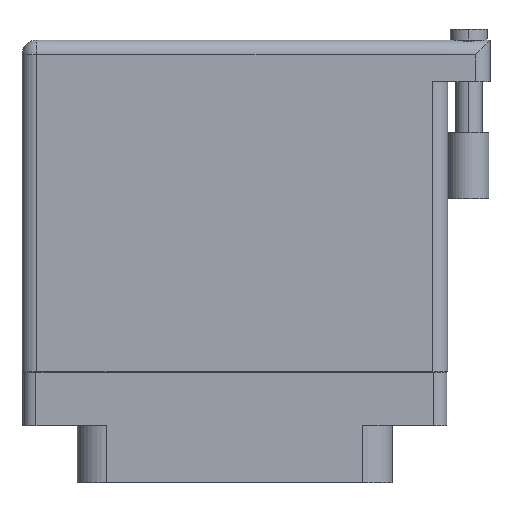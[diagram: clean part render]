
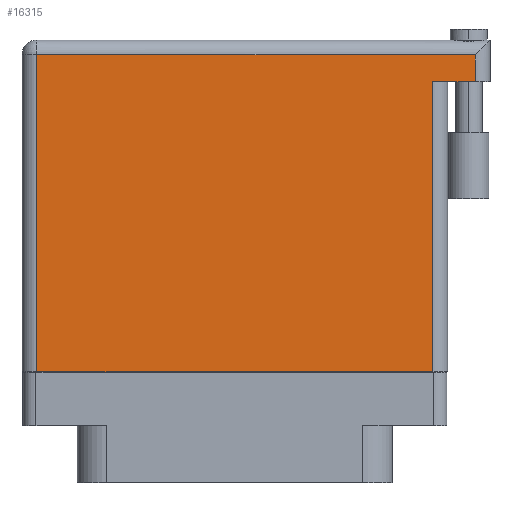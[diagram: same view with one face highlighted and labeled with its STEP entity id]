
A CAD part, front view. The second image highlights one B-rep face of the part: STEP entity #16315.
In plain terms, the highlighted face is planar.
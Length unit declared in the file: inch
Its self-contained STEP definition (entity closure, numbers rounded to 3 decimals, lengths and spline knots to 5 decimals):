
#900 = EDGE_CURVE ( 'NONE', #13234, #25031, #27384, .T. ) ;
#1510 = CARTESIAN_POINT ( 'NONE',  ( -0.934, 1.396, 0.4495 ) ) ;
#2189 = CARTESIAN_POINT ( 'NONE',  ( -1.004, -0.1, 0.4495 ) ) ;
#2897 = PLANE ( 'NONE',  #20986 ) ;
#4663 = DIRECTION ( 'NONE',  ( 1., 0., 0. ) ) ;
#4667 = CARTESIAN_POINT ( 'NONE',  ( 0.934, 1.269, 0.4495 ) ) ;
#4809 = ORIENTED_EDGE ( 'NONE', *, *, #14126, .T. ) ;
#5368 = DIRECTION ( 'NONE',  ( -1., 0., 0. ) ) ;
#5588 = VECTOR ( 'NONE', #29237, 39.37008 ) ;
#5783 = VECTOR ( 'NONE', #17002, 39.37008 ) ;
#6288 = VECTOR ( 'NONE', #26266, 39.37008 ) ;
#7464 = CARTESIAN_POINT ( 'NONE',  ( 1.134, 1.396, 0.4495 ) ) ;
#7472 = VECTOR ( 'NONE', #4663, 39.37008 ) ;
#8969 = CARTESIAN_POINT ( 'NONE',  ( -1.004, 1.396, 0.4495 ) ) ;
#9119 = VECTOR ( 'NONE', #24886, 39.37008 ) ;
#9122 = ORIENTED_EDGE ( 'NONE', *, *, #14256, .T. ) ;
#10076 = ORIENTED_EDGE ( 'NONE', *, *, #21567, .T. ) ;
#10309 = CARTESIAN_POINT ( 'NONE',  ( -1.004, 1.466, 0.4495 ) ) ;
#10380 = LINE ( 'NONE', #26793, #5783 ) ;
#10939 = VERTEX_POINT ( 'NONE', #24874 ) ;
#12485 = CARTESIAN_POINT ( 'NONE',  ( -0.934, -0.1, 0.4495 ) ) ;
#13234 = VERTEX_POINT ( 'NONE', #7464 ) ;
#13958 = VECTOR ( 'NONE', #24196, 39.37008 ) ;
#14126 = EDGE_CURVE ( 'NONE', #10939, #17827, #21335, .T. ) ;
#14256 = EDGE_CURVE ( 'NONE', #17827, #18889, #30117, .T. ) ;
#15545 = ORIENTED_EDGE ( 'NONE', *, *, #23835, .F. ) ;
#16315 = ADVANCED_FACE ( 'NONE', ( #23853 ), #2897, .F. ) ;
#17002 = DIRECTION ( 'NONE',  ( 0., 1., 0. ) ) ;
#17118 = ORIENTED_EDGE ( 'NONE', *, *, #900, .T. ) ;
#17488 = LINE ( 'NONE', #12485, #5588 ) ;
#17827 = VERTEX_POINT ( 'NONE', #19829 ) ;
#18889 = VERTEX_POINT ( 'NONE', #4667 ) ;
#19829 = CARTESIAN_POINT ( 'NONE',  ( 0.934, -0.1, 0.4495 ) ) ;
#20360 = CARTESIAN_POINT ( 'NONE',  ( 1.204, 1.269, 0.4495 ) ) ;
#20986 = AXIS2_PLACEMENT_3D ( 'NONE', #10309, #22451, #5368 ) ;
#21335 = LINE ( 'NONE', #2189, #7472 ) ;
#21567 = EDGE_CURVE ( 'NONE', #28673, #13234, #10380, .T. ) ;
#22451 = DIRECTION ( 'NONE',  ( 0., 0., -1. ) ) ;
#23075 = ORIENTED_EDGE ( 'NONE', *, *, #27894, .T. ) ;
#23835 = EDGE_CURVE ( 'NONE', #28673, #18889, #24491, .T. ) ;
#23853 = FACE_OUTER_BOUND ( 'NONE', #27603, .T. ) ;
#24196 = DIRECTION ( 'NONE',  ( 0., 1., 0. ) ) ;
#24491 = LINE ( 'NONE', #20360, #9119 ) ;
#24874 = CARTESIAN_POINT ( 'NONE',  ( -0.934, -0.1, 0.4495 ) ) ;
#24886 = DIRECTION ( 'NONE',  ( -1., 0., 0. ) ) ;
#25031 = VERTEX_POINT ( 'NONE', #1510 ) ;
#26266 = DIRECTION ( 'NONE',  ( -1., 0., 0. ) ) ;
#26793 = CARTESIAN_POINT ( 'NONE',  ( 1.134, 1.466, 0.4495 ) ) ;
#27384 = LINE ( 'NONE', #8969, #6288 ) ;
#27603 = EDGE_LOOP ( 'NONE', ( #4809, #9122, #15545, #10076, #17118, #23075 ) ) ;
#27894 = EDGE_CURVE ( 'NONE', #25031, #10939, #17488, .T. ) ;
#28673 = VERTEX_POINT ( 'NONE', #31136 ) ;
#29237 = DIRECTION ( 'NONE',  ( 0., -1., 0. ) ) ;
#30117 = LINE ( 'NONE', #31407, #13958 ) ;
#31136 = CARTESIAN_POINT ( 'NONE',  ( 1.134, 1.269, 0.4495 ) ) ;
#31407 = CARTESIAN_POINT ( 'NONE',  ( 0.934, 1.269, 0.4495 ) ) ;
